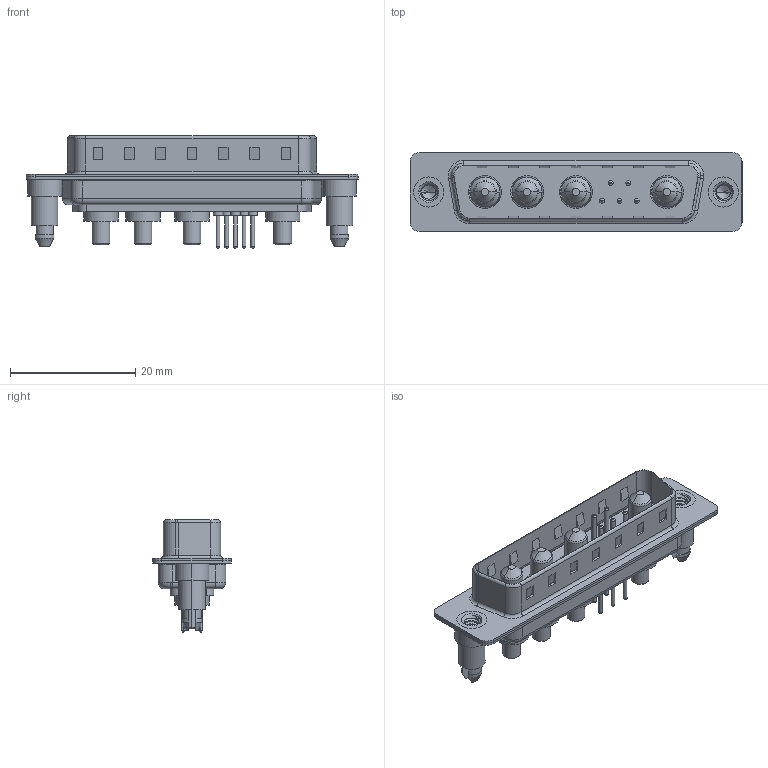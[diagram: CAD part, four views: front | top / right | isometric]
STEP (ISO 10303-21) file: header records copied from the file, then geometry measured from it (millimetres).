
FILE_DESCRIPTION (( 'STEP AP203' ), '1' );
FILE_NAME ('627-9W4-624-2T5.STEP', '2019-05-26T09:09:55', ( '' ), ( '' ), 'SwSTEP 2.0', 'SolidWorks 2016', '' );
FILE_SCHEMA (( 'CONFIG_CONTROL_DESIGN' ));
Length unit declared in the file: millimetre
Products named in the file (8): 627Combo Housing_9W4; 627Combo Shell Rear_25 Contacts; 627Combo Shell Front_25 Contacts; 627Combo Threaded Boardlock_5; Power Pin_20A S; 627Combo Contact Row 1_24; 627Combo Contact Row 2_24; 627-9W4-624-2T5
Assembly tree (14 placements, depth 2):
  627-9W4-624-2T5
    627Combo Housing_9W4
    627Combo Shell Rear_25 Contacts
    627Combo Shell Front_25 Contacts
    627Combo Threaded Boardlock_5  x2
    Power Pin_20A S  x4
    627Combo Contact Row 1_24  x2
    627Combo Contact Row 2_24  x3
Bounding box: 53 x 12.6 x 17.9 mm (x, y, z)
Volume: 3127.6 mm3; surface area: 7042.9 mm2
Topology: 18 solids, 18 shells, 771 faces, 1799 edges, 1116 vertices
Faces by surface type: cylinder 315, plane 262, torus 138, cone 42, bspline 14
Entity records: 18029 total; most frequent: CARTESIAN_POINT 4410, DIRECTION 2780, ORIENTED_EDGE 2522, EDGE_CURVE 1261, AXIS2_PLACEMENT_3D 1062, VERTEX_POINT 793, VECTOR 656, LINE 656
